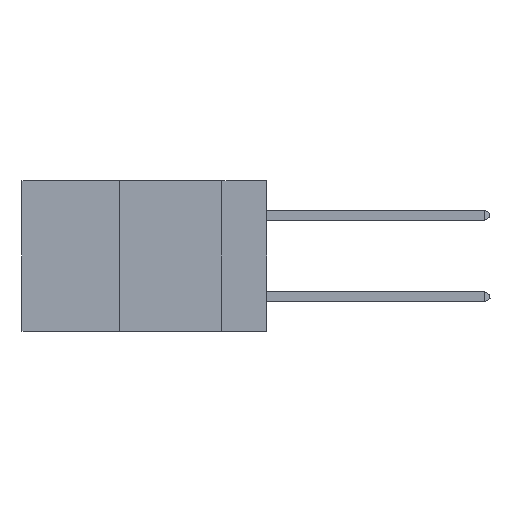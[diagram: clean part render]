
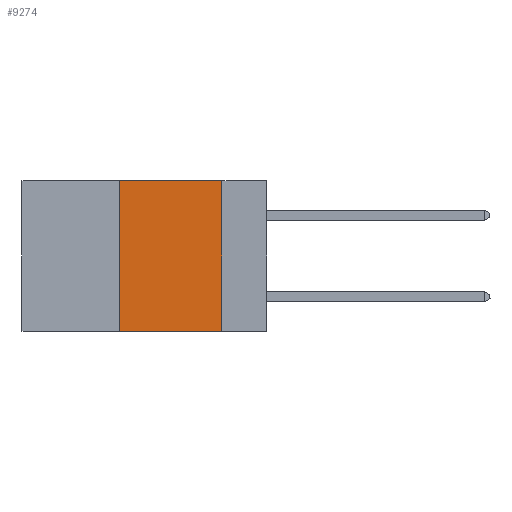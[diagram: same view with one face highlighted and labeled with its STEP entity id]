
A CAD part, left-side view. The second image highlights one B-rep face of the part: STEP entity #9274.
In plain terms, the highlighted planar face has unit normal (-1, 0, 0).
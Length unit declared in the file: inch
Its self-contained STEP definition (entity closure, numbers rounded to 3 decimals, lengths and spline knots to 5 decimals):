
#9 = VERTEX_POINT ( 'NONE', #6087 ) ;
#114 = EDGE_CURVE ( 'NONE', #8679, #6321, #1045, .T. ) ;
#292 = EDGE_CURVE ( 'NONE', #9028, #9, #2011, .T. ) ;
#828 = CARTESIAN_POINT ( 'NONE',  ( 0., 0.11, 0. ) ) ;
#865 = FACE_OUTER_BOUND ( 'NONE', #2337, .T. ) ;
#1045 = LINE ( 'NONE', #2444, #3572 ) ;
#1121 = DIRECTION ( 'NONE',  ( 0., 0., -1. ) ) ;
#1749 = DIRECTION ( 'NONE',  ( 0., -1., 0. ) ) ;
#2011 = LINE ( 'NONE', #828, #9908 ) ;
#2337 = EDGE_LOOP ( 'NONE', ( #5396, #7371, #7777, #4469 ) ) ;
#2444 = CARTESIAN_POINT ( 'NONE',  ( 0., 0.36, 0. ) ) ;
#2946 = EDGE_CURVE ( 'NONE', #8679, #9, #8868, .T. ) ;
#2966 = DIRECTION ( 'NONE',  ( 0., 0., 1. ) ) ;
#3572 = VECTOR ( 'NONE', #2966, 39.37008 ) ;
#3856 = AXIS2_PLACEMENT_3D ( 'NONE', #4791, #9997, #5595 ) ;
#3995 = PLANE ( 'NONE',  #3856 ) ;
#4469 = ORIENTED_EDGE ( 'NONE', *, *, #2946, .T. ) ;
#4791 = CARTESIAN_POINT ( 'NONE',  ( 0., 0.6, 0. ) ) ;
#5227 = LINE ( 'NONE', #8743, #7022 ) ;
#5240 = EDGE_CURVE ( 'NONE', #6321, #9028, #5227, .T. ) ;
#5396 = ORIENTED_EDGE ( 'NONE', *, *, #292, .F. ) ;
#5595 = DIRECTION ( 'NONE',  ( 0., 0., -1. ) ) ;
#6048 = CARTESIAN_POINT ( 'NONE',  ( 0., 0.11, 0. ) ) ;
#6087 = CARTESIAN_POINT ( 'NONE',  ( 0., 0.11, -0.37 ) ) ;
#6321 = VERTEX_POINT ( 'NONE', #7154 ) ;
#6931 = VECTOR ( 'NONE', #1749, 39.37008 ) ;
#7022 = VECTOR ( 'NONE', #9472, 39.37008 ) ;
#7069 = CARTESIAN_POINT ( 'NONE',  ( 0., 0.6, -0.37 ) ) ;
#7154 = CARTESIAN_POINT ( 'NONE',  ( 0., 0.36, 0. ) ) ;
#7371 = ORIENTED_EDGE ( 'NONE', *, *, #5240, .F. ) ;
#7777 = ORIENTED_EDGE ( 'NONE', *, *, #114, .F. ) ;
#8395 = CARTESIAN_POINT ( 'NONE',  ( 0., 0.36, -0.37 ) ) ;
#8679 = VERTEX_POINT ( 'NONE', #8395 ) ;
#8743 = CARTESIAN_POINT ( 'NONE',  ( 0., 0.6, 0. ) ) ;
#8868 = LINE ( 'NONE', #7069, #6931 ) ;
#9028 = VERTEX_POINT ( 'NONE', #6048 ) ;
#9274 = ADVANCED_FACE ( 'NONE', ( #865 ), #3995, .F. ) ;
#9472 = DIRECTION ( 'NONE',  ( 0., -1., 0. ) ) ;
#9908 = VECTOR ( 'NONE', #1121, 39.37008 ) ;
#9997 = DIRECTION ( 'NONE',  ( 1., 0., 0. ) ) ;
